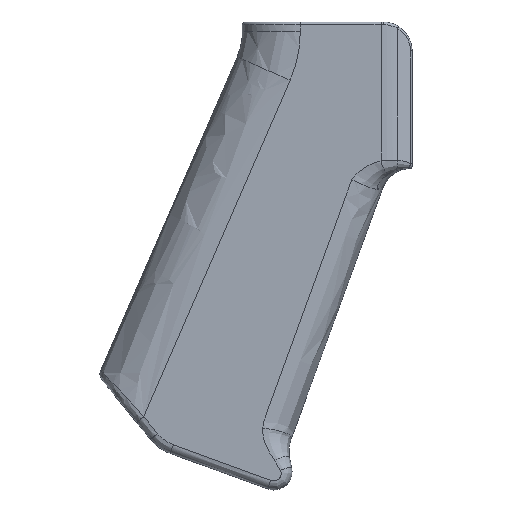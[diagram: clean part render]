
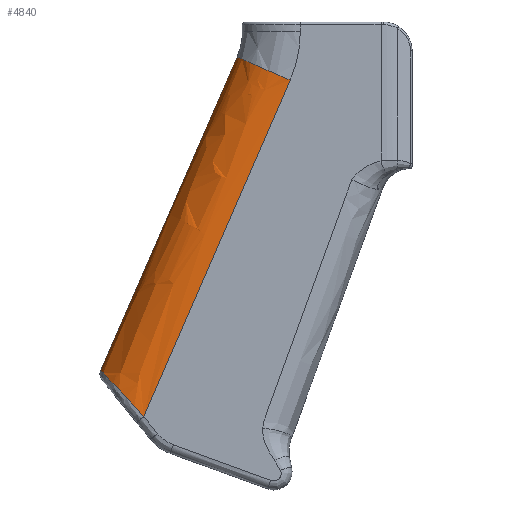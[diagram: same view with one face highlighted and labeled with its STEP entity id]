
A CAD part, left-side view. The second image highlights one B-rep face of the part: STEP entity #4840.
In plain terms, the highlighted free-form (B-spline) face has degree [1, 2] with [2, 3] control points.
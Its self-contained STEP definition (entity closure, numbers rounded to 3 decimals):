
#30=(
BOUNDED_SURFACE()
B_SPLINE_SURFACE(1,2,((#11365,#11366,#11367),(#11368,#11369,#11370)),
 .UNSPECIFIED.,.F.,.F.,.F.)
B_SPLINE_SURFACE_WITH_KNOTS((2,2),(3,3),(0.,6.338),
(-1.571,0.),.UNSPECIFIED.)
GEOMETRIC_REPRESENTATION_ITEM()
RATIONAL_B_SPLINE_SURFACE(((1.,0.707,1.),(1.,0.707,
1.)))
REPRESENTATION_ITEM('')
SURFACE()
);
#44=ELLIPSE('',#5099,12.692,11.);
#397=B_SPLINE_CURVE_WITH_KNOTS('',3,(#11043,#11044,#11045,#11046,#11047,
#11048,#11049),.UNSPECIFIED.,.F.,.F.,(4,1,1,1,4),(-1.675,-0.964,
-0.49,-0.253,-0.016),
 .UNSPECIFIED.);
#771=FACE_OUTER_BOUND('',#1058,.T.);
#1058=EDGE_LOOP('',(#4393,#4394,#4395,#4396));
#1440=LINE('',#10325,#1834);
#1452=LINE('',#11363,#1846);
#1834=VECTOR('',#5916,10.);
#1846=VECTOR('',#5952,10.);
#2286=VERTEX_POINT('',#10322);
#2287=VERTEX_POINT('',#10324);
#2300=VERTEX_POINT('',#10977);
#2306=VERTEX_POINT('',#11362);
#2967=EDGE_CURVE('',#2287,#2286,#1440,.T.);
#2992=EDGE_CURVE('',#2287,#2300,#397,.T.);
#3008=EDGE_CURVE('',#2300,#2306,#1452,.T.);
#3010=EDGE_CURVE('',#2306,#2286,#44,.T.);
#4393=ORIENTED_EDGE('',*,*,#2992,.F.);
#4394=ORIENTED_EDGE('',*,*,#2967,.T.);
#4395=ORIENTED_EDGE('',*,*,#3010,.F.);
#4396=ORIENTED_EDGE('',*,*,#3008,.F.);
#4840=ADVANCED_FACE('',(#771),#30,.F.);
#5099=AXIS2_PLACEMENT_3D('',#11371,#5954,#5955);
#5916=DIRECTION('',(0.,-0.399,0.917));
#5952=DIRECTION('',(0.,-0.399,0.917));
#5954=DIRECTION('center_axis',(0.,-0.399,
0.917));
#5955=DIRECTION('ref_axis',(0.,0.917,0.399));
#10322=CARTESIAN_POINT('',(-11.49,-127.561,-21.956));
#10324=CARTESIAN_POINT('',(-11.49,-95.456,-95.713));
#10325=CARTESIAN_POINT('',(-11.49,-127.561,-21.956));
#10977=CARTESIAN_POINT('',(-0.49,-86.02,-85.59));
#11043=CARTESIAN_POINT('Ctrl Pts',(-11.49,-95.456,
-95.713));
#11044=CARTESIAN_POINT('Ctrl Pts',(-11.49,-93.653,
-93.743));
#11045=CARTESIAN_POINT('Ctrl Pts',(-10.515,-90.631,
-90.442));
#11046=CARTESIAN_POINT('Ctrl Pts',(-6.963,-87.569,
-87.189));
#11047=CARTESIAN_POINT('Ctrl Pts',(-3.486,-86.263,
-85.838));
#11048=CARTESIAN_POINT('Ctrl Pts',(-1.489,-86.02,
-85.59));
#11049=CARTESIAN_POINT('Ctrl Pts',(-0.49,-86.02,
-85.59));
#11362=CARTESIAN_POINT('',(-0.49,-115.924,-16.89));
#11363=CARTESIAN_POINT('',(-0.49,-115.924,-16.89));
#11365=CARTESIAN_POINT('Ctrl Pts',(-11.49,-127.561,
-21.956));
#11366=CARTESIAN_POINT('Ctrl Pts',(-11.49,-115.924,-16.89));
#11367=CARTESIAN_POINT('Ctrl Pts',(-0.49,-115.924,-16.89));
#11368=CARTESIAN_POINT('Ctrl Pts',(-11.49,-95.456,-95.713));
#11369=CARTESIAN_POINT('Ctrl Pts',(-11.49,-83.819,
-90.648));
#11370=CARTESIAN_POINT('Ctrl Pts',(-0.49,-83.819,
-90.648));
#11371=CARTESIAN_POINT('Origin',(-0.49,-127.561,-21.956));
